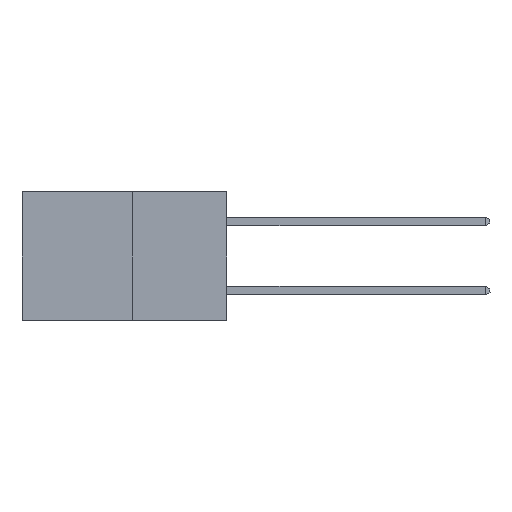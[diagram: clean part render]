
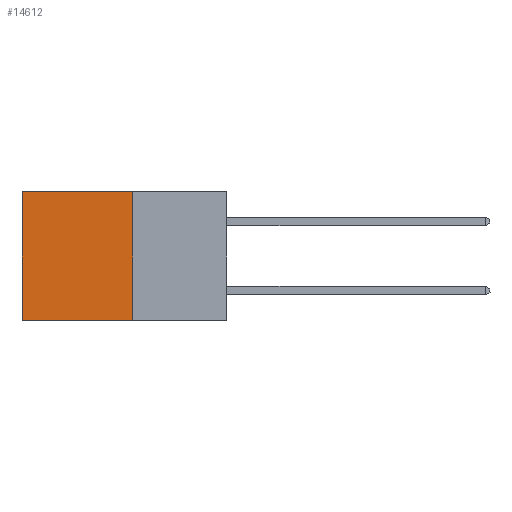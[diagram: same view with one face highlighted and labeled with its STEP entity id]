
A CAD part, left-side view. The second image highlights one B-rep face of the part: STEP entity #14612.
In plain terms, the highlighted planar face has unit normal (-1, 0, 0).
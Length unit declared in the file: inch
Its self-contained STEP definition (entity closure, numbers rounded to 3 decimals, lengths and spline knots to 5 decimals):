
#256 = LINE ( 'NONE', #3079, #17702 ) ;
#2421 = DIRECTION ( 'NONE',  ( 1., 0., 0. ) ) ;
#3079 = CARTESIAN_POINT ( 'NONE',  ( 0.277, 0.59, -0.37 ) ) ;
#3151 = ORIENTED_EDGE ( 'NONE', *, *, #18799, .T. ) ;
#3314 = VERTEX_POINT ( 'NONE', #6494 ) ;
#3412 = VECTOR ( 'NONE', #20295, 39.37008 ) ;
#4484 = DIRECTION ( 'NONE',  ( 0., 0., -1. ) ) ;
#4660 = AXIS2_PLACEMENT_3D ( 'NONE', #14198, #2421, #14263 ) ;
#4725 = CARTESIAN_POINT ( 'NONE',  ( 0.277, 0.27, -0.37 ) ) ;
#6025 = ORIENTED_EDGE ( 'NONE', *, *, #6561, .F. ) ;
#6494 = CARTESIAN_POINT ( 'NONE',  ( 0.277, 0.59, -0.37 ) ) ;
#6561 = EDGE_CURVE ( 'NONE', #14779, #14225, #15132, .T. ) ;
#7607 = EDGE_LOOP ( 'NONE', ( #15217, #18281, #6025, #3151 ) ) ;
#8152 = EDGE_CURVE ( 'NONE', #14225, #3314, #21240, .T. ) ;
#8411 = VERTEX_POINT ( 'NONE', #17983 ) ;
#8689 = CARTESIAN_POINT ( 'NONE',  ( 0.277, 0.27, 0. ) ) ;
#10871 = PLANE ( 'NONE',  #4660 ) ;
#12145 = VECTOR ( 'NONE', #17065, 39.37008 ) ;
#12246 = CARTESIAN_POINT ( 'NONE',  ( 0.277, 0.27, 0. ) ) ;
#14198 = CARTESIAN_POINT ( 'NONE',  ( 0.277, 0.27, -0.37 ) ) ;
#14225 = VERTEX_POINT ( 'NONE', #19647 ) ;
#14263 = DIRECTION ( 'NONE',  ( 0., 0., -1. ) ) ;
#14612 = ADVANCED_FACE ( 'NONE', ( #16460 ), #10871, .F. ) ;
#14779 = VERTEX_POINT ( 'NONE', #12246 ) ;
#15132 = LINE ( 'NONE', #4725, #20063 ) ;
#15184 = EDGE_CURVE ( 'NONE', #8411, #3314, #256, .T. ) ;
#15217 = ORIENTED_EDGE ( 'NONE', *, *, #15184, .T. ) ;
#16460 = FACE_OUTER_BOUND ( 'NONE', #7607, .T. ) ;
#16596 = DIRECTION ( 'NONE',  ( 0., 0., -1. ) ) ;
#17065 = DIRECTION ( 'NONE',  ( 0., 1., 0. ) ) ;
#17702 = VECTOR ( 'NONE', #16596, 39.37008 ) ;
#17983 = CARTESIAN_POINT ( 'NONE',  ( 0.277, 0.59, 0. ) ) ;
#18281 = ORIENTED_EDGE ( 'NONE', *, *, #8152, .F. ) ;
#18564 = CARTESIAN_POINT ( 'NONE',  ( 0.277, 0.27, -0.37 ) ) ;
#18799 = EDGE_CURVE ( 'NONE', #14779, #8411, #21502, .T. ) ;
#19647 = CARTESIAN_POINT ( 'NONE',  ( 0.277, 0.27, -0.37 ) ) ;
#20063 = VECTOR ( 'NONE', #4484, 39.37008 ) ;
#20295 = DIRECTION ( 'NONE',  ( 0., 1., 0. ) ) ;
#21240 = LINE ( 'NONE', #18564, #3412 ) ;
#21502 = LINE ( 'NONE', #8689, #12145 ) ;
